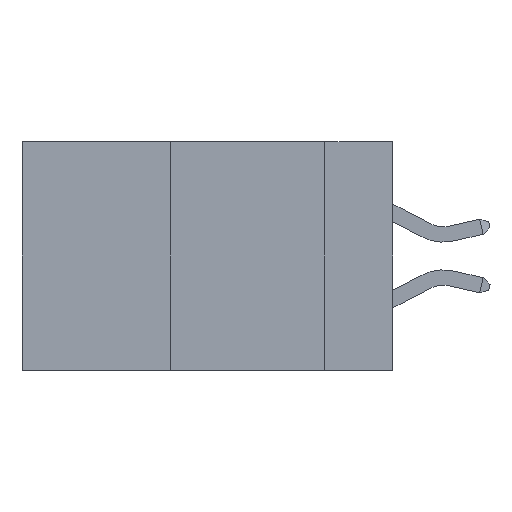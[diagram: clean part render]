
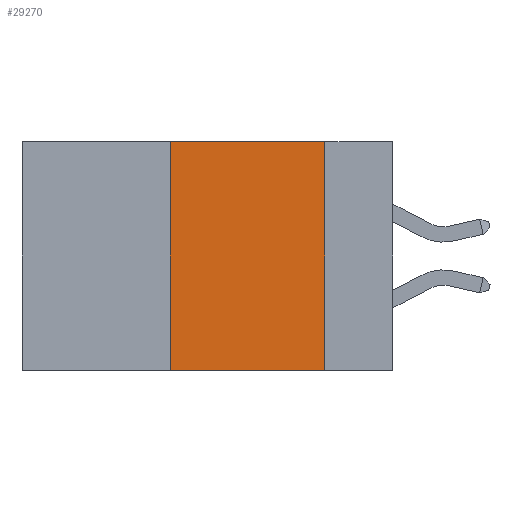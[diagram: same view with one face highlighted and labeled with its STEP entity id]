
A CAD part, left-side view. The second image highlights one B-rep face of the part: STEP entity #29270.
In plain terms, the highlighted planar face has unit normal (-1, 0, 0).
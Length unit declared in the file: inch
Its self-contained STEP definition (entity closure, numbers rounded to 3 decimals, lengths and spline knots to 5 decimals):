
#1170 = VERTEX_POINT ( 'NONE', #32017 ) ;
#1481 = LINE ( 'NONE', #18074, #27697 ) ;
#2239 = CARTESIAN_POINT ( 'NONE',  ( 0., 0.6, 0. ) ) ;
#3306 = AXIS2_PLACEMENT_3D ( 'NONE', #19928, #16928, #25201 ) ;
#5313 = VECTOR ( 'NONE', #18027, 39.37008 ) ;
#5452 = LINE ( 'NONE', #15642, #27997 ) ;
#6700 = LINE ( 'NONE', #23127, #16502 ) ;
#7993 = DIRECTION ( 'NONE',  ( 0., -1., 0. ) ) ;
#8478 = VERTEX_POINT ( 'NONE', #15493 ) ;
#10216 = LINE ( 'NONE', #2239, #5313 ) ;
#10666 = CARTESIAN_POINT ( 'NONE',  ( 0., 0.11, -0.37 ) ) ;
#12675 = CARTESIAN_POINT ( 'NONE',  ( 0., 0.36, -0.37 ) ) ;
#13115 = ORIENTED_EDGE ( 'NONE', *, *, #32828, .F. ) ;
#13872 = FACE_OUTER_BOUND ( 'NONE', #33830, .T. ) ;
#15493 = CARTESIAN_POINT ( 'NONE',  ( 0., 0.11, 0. ) ) ;
#15642 = CARTESIAN_POINT ( 'NONE',  ( 0., 0.6, -0.37 ) ) ;
#16502 = VECTOR ( 'NONE', #22222, 39.37008 ) ;
#16928 = DIRECTION ( 'NONE',  ( 1., 0., 0. ) ) ;
#17271 = PLANE ( 'NONE',  #3306 ) ;
#17579 = EDGE_CURVE ( 'NONE', #8478, #32990, #6700, .T. ) ;
#17605 = ORIENTED_EDGE ( 'NONE', *, *, #17579, .F. ) ;
#18027 = DIRECTION ( 'NONE',  ( 0., -1., 0. ) ) ;
#18074 = CARTESIAN_POINT ( 'NONE',  ( 0., 0.36, 0. ) ) ;
#19539 = EDGE_CURVE ( 'NONE', #27488, #1170, #1481, .T. ) ;
#19928 = CARTESIAN_POINT ( 'NONE',  ( 0., 0.6, 0. ) ) ;
#22222 = DIRECTION ( 'NONE',  ( 0., 0., -1. ) ) ;
#23127 = CARTESIAN_POINT ( 'NONE',  ( 0., 0.11, 0. ) ) ;
#25201 = DIRECTION ( 'NONE',  ( 0., 0., -1. ) ) ;
#27488 = VERTEX_POINT ( 'NONE', #12675 ) ;
#27676 = EDGE_CURVE ( 'NONE', #27488, #32990, #5452, .T. ) ;
#27697 = VECTOR ( 'NONE', #31568, 39.37008 ) ;
#27891 = ORIENTED_EDGE ( 'NONE', *, *, #19539, .F. ) ;
#27997 = VECTOR ( 'NONE', #7993, 39.37008 ) ;
#29270 = ADVANCED_FACE ( 'NONE', ( #13872 ), #17271, .F. ) ;
#29538 = ORIENTED_EDGE ( 'NONE', *, *, #27676, .T. ) ;
#31568 = DIRECTION ( 'NONE',  ( 0., 0., 1. ) ) ;
#32017 = CARTESIAN_POINT ( 'NONE',  ( 0., 0.36, 0. ) ) ;
#32828 = EDGE_CURVE ( 'NONE', #1170, #8478, #10216, .T. ) ;
#32990 = VERTEX_POINT ( 'NONE', #10666 ) ;
#33830 = EDGE_LOOP ( 'NONE', ( #17605, #13115, #27891, #29538 ) ) ;
